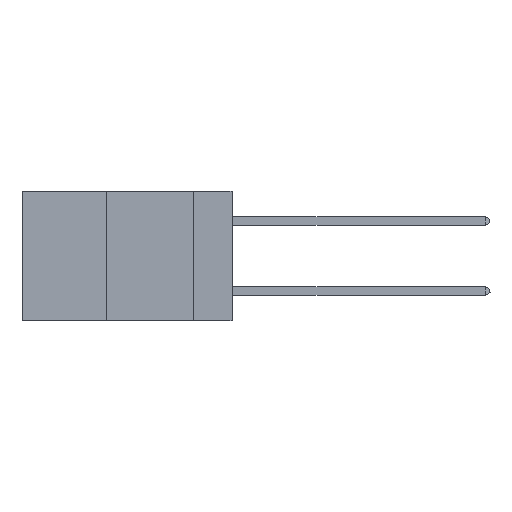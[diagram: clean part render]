
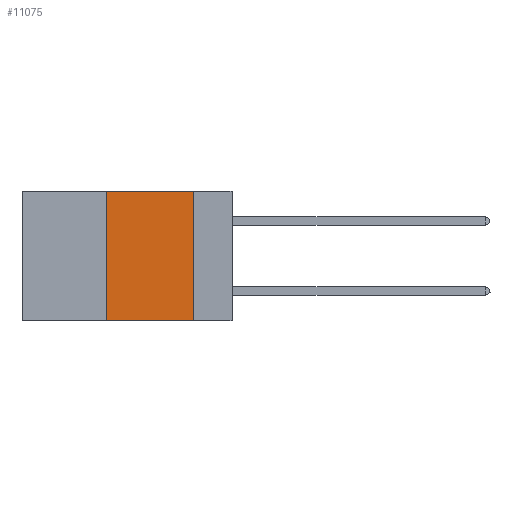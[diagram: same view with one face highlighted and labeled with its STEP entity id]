
A CAD part, left-side view. The second image highlights one B-rep face of the part: STEP entity #11075.
In plain terms, the highlighted planar face has unit normal (-1, 0, 0).
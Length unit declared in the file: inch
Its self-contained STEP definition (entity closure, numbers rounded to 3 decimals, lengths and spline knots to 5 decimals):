
#144 = EDGE_CURVE ( 'NONE', #15923, #10864, #12492, .T. ) ;
#311 = CARTESIAN_POINT ( 'NONE',  ( 0., 0.6, 0. ) ) ;
#588 = EDGE_CURVE ( 'NONE', #7637, #8658, #4081, .T. ) ;
#951 = LINE ( 'NONE', #4049, #13330 ) ;
#1470 = DIRECTION ( 'NONE',  ( 0., 0., -1. ) ) ;
#2651 = DIRECTION ( 'NONE',  ( 1., 0., 0. ) ) ;
#3292 = CARTESIAN_POINT ( 'NONE',  ( 0., 0.36, -0.37 ) ) ;
#3314 = CARTESIAN_POINT ( 'NONE',  ( 0., 0.11, 0. ) ) ;
#3692 = ORIENTED_EDGE ( 'NONE', *, *, #13210, .F. ) ;
#4049 = CARTESIAN_POINT ( 'NONE',  ( 0., 0.6, -0.37 ) ) ;
#4081 = LINE ( 'NONE', #11545, #13626 ) ;
#4181 = VECTOR ( 'NONE', #14711, 39.37008 ) ;
#5322 = DIRECTION ( 'NONE',  ( 0., -1., 0. ) ) ;
#5378 = PLANE ( 'NONE',  #15893 ) ;
#6011 = ORIENTED_EDGE ( 'NONE', *, *, #144, .F. ) ;
#7435 = VECTOR ( 'NONE', #9595, 39.37008 ) ;
#7637 = VERTEX_POINT ( 'NONE', #3292 ) ;
#8542 = CARTESIAN_POINT ( 'NONE',  ( 0., 0.6, 0. ) ) ;
#8655 = CARTESIAN_POINT ( 'NONE',  ( 0., 0.11, -0.37 ) ) ;
#8658 = VERTEX_POINT ( 'NONE', #13878 ) ;
#8846 = DIRECTION ( 'NONE',  ( 0., 0., 1. ) ) ;
#9595 = DIRECTION ( 'NONE',  ( 0., 0., -1. ) ) ;
#10719 = ORIENTED_EDGE ( 'NONE', *, *, #588, .F. ) ;
#10864 = VERTEX_POINT ( 'NONE', #8655 ) ;
#11075 = ADVANCED_FACE ( 'NONE', ( #11988 ), #5378, .F. ) ;
#11450 = EDGE_LOOP ( 'NONE', ( #6011, #3692, #10719, #13243 ) ) ;
#11545 = CARTESIAN_POINT ( 'NONE',  ( 0., 0.36, 0. ) ) ;
#11988 = FACE_OUTER_BOUND ( 'NONE', #11450, .T. ) ;
#12230 = CARTESIAN_POINT ( 'NONE',  ( 0., 0.11, 0. ) ) ;
#12492 = LINE ( 'NONE', #3314, #7435 ) ;
#13210 = EDGE_CURVE ( 'NONE', #8658, #15923, #14696, .T. ) ;
#13243 = ORIENTED_EDGE ( 'NONE', *, *, #14038, .T. ) ;
#13330 = VECTOR ( 'NONE', #5322, 39.37008 ) ;
#13626 = VECTOR ( 'NONE', #8846, 39.37008 ) ;
#13878 = CARTESIAN_POINT ( 'NONE',  ( 0., 0.36, 0. ) ) ;
#14038 = EDGE_CURVE ( 'NONE', #7637, #10864, #951, .T. ) ;
#14696 = LINE ( 'NONE', #8542, #4181 ) ;
#14711 = DIRECTION ( 'NONE',  ( 0., -1., 0. ) ) ;
#15893 = AXIS2_PLACEMENT_3D ( 'NONE', #311, #2651, #1470 ) ;
#15923 = VERTEX_POINT ( 'NONE', #12230 ) ;
